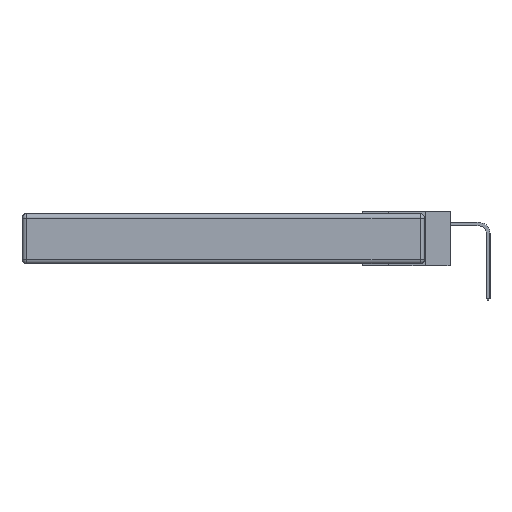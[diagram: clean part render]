
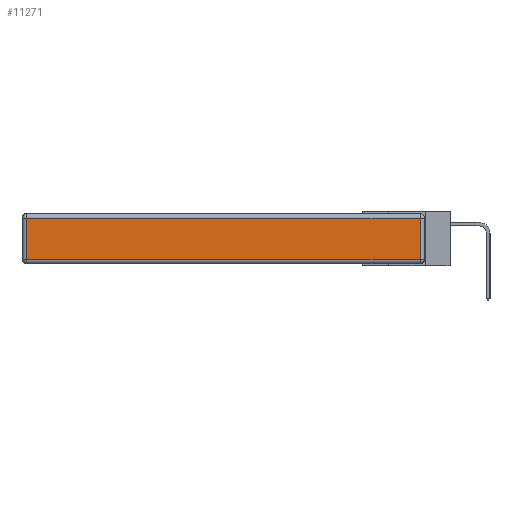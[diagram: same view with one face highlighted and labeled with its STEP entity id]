
A CAD part, left-side view. The second image highlights one B-rep face of the part: STEP entity #11271.
In plain terms, the highlighted planar face has unit normal (-1, 0, 0).
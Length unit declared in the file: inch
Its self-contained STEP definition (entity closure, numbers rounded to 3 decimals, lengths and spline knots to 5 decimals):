
#511 = PLANE ( 'NONE',  #14618 ) ;
#1356 = CARTESIAN_POINT ( 'NONE',  ( 0., 0.03, -0.03 ) ) ;
#2314 = LINE ( 'NONE', #9098, #5467 ) ;
#2527 = FACE_OUTER_BOUND ( 'NONE', #13537, .T. ) ;
#4351 = EDGE_CURVE ( 'NONE', #15903, #14741, #10630, .T. ) ;
#5467 = VECTOR ( 'NONE', #7343, 39.37008 ) ;
#5506 = CARTESIAN_POINT ( 'NONE',  ( 0., 2.75, -0.03 ) ) ;
#5543 = CARTESIAN_POINT ( 'NONE',  ( 0., 0., -0.343 ) ) ;
#5783 = CARTESIAN_POINT ( 'NONE',  ( 0., 0., -0.313 ) ) ;
#5910 = EDGE_CURVE ( 'NONE', #20960, #15903, #19058, .T. ) ;
#6280 = LINE ( 'NONE', #5506, #17125 ) ;
#7343 = DIRECTION ( 'NONE',  ( 0., 0., -1. ) ) ;
#9098 = CARTESIAN_POINT ( 'NONE',  ( 0., 2.72, -0.343 ) ) ;
#9602 = VERTEX_POINT ( 'NONE', #15301 ) ;
#10630 = LINE ( 'NONE', #18418, #18326 ) ;
#10878 = DIRECTION ( 'NONE',  ( 0., -1., 0. ) ) ;
#11271 = ADVANCED_FACE ( 'NONE', ( #2527 ), #511, .T. ) ;
#11672 = ORIENTED_EDGE ( 'NONE', *, *, #5910, .T. ) ;
#12112 = DIRECTION ( 'NONE',  ( 0., 1., 0. ) ) ;
#12162 = CARTESIAN_POINT ( 'NONE',  ( 0., 2.72, -0.313 ) ) ;
#12189 = ORIENTED_EDGE ( 'NONE', *, *, #15644, .T. ) ;
#13537 = EDGE_LOOP ( 'NONE', ( #11672, #16430, #12189, #15663 ) ) ;
#13972 = DIRECTION ( 'NONE',  ( -1., 0., 0. ) ) ;
#14618 = AXIS2_PLACEMENT_3D ( 'NONE', #5543, #13972, #18867 ) ;
#14741 = VERTEX_POINT ( 'NONE', #1356 ) ;
#15301 = CARTESIAN_POINT ( 'NONE',  ( 0., 2.72, -0.03 ) ) ;
#15644 = EDGE_CURVE ( 'NONE', #14741, #9602, #6280, .T. ) ;
#15663 = ORIENTED_EDGE ( 'NONE', *, *, #17937, .T. ) ;
#15903 = VERTEX_POINT ( 'NONE', #21205 ) ;
#16430 = ORIENTED_EDGE ( 'NONE', *, *, #4351, .T. ) ;
#16553 = DIRECTION ( 'NONE',  ( 0., 0., 1. ) ) ;
#17125 = VECTOR ( 'NONE', #12112, 39.37008 ) ;
#17937 = EDGE_CURVE ( 'NONE', #9602, #20960, #2314, .T. ) ;
#18275 = VECTOR ( 'NONE', #10878, 39.37008 ) ;
#18326 = VECTOR ( 'NONE', #16553, 39.37008 ) ;
#18418 = CARTESIAN_POINT ( 'NONE',  ( 0., 0.03, -0.343 ) ) ;
#18867 = DIRECTION ( 'NONE',  ( 0., 0., 1. ) ) ;
#19058 = LINE ( 'NONE', #5783, #18275 ) ;
#20960 = VERTEX_POINT ( 'NONE', #12162 ) ;
#21205 = CARTESIAN_POINT ( 'NONE',  ( 0., 0.03, -0.313 ) ) ;
